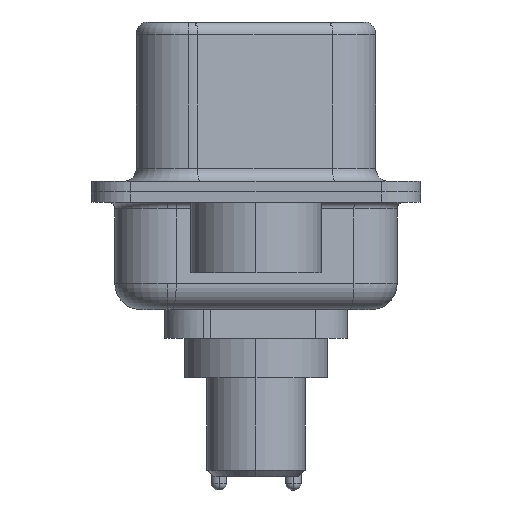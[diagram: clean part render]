
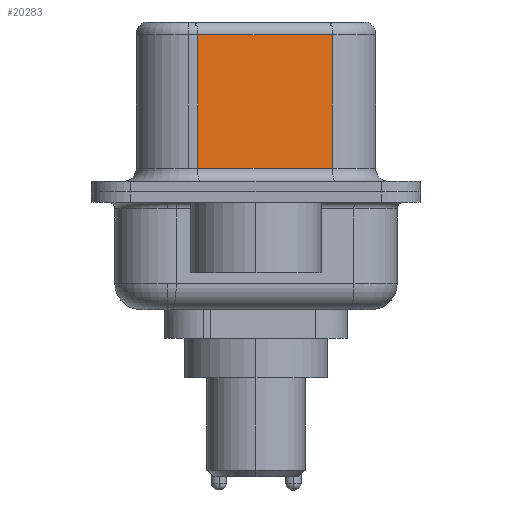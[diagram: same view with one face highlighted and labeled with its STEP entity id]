
A CAD part, left-side view. The second image highlights one B-rep face of the part: STEP entity #20283.
In plain terms, the highlighted planar face has unit normal (-0.985, -0.174, 0).
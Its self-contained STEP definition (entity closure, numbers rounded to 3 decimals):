
#166 = DIRECTION ( 'NONE',  ( 0., 0., -1. ) ) ;
#474 = VERTEX_POINT ( 'NONE', #5944 ) ;
#1858 = EDGE_CURVE ( 'NONE', #18986, #15144, #6978, .T. ) ;
#3460 = LINE ( 'NONE', #5739, #17208 ) ;
#3616 = DIRECTION ( 'NONE',  ( -0.174, 0.985, 0. ) ) ;
#3842 = VECTOR ( 'NONE', #9684, 1000. ) ;
#4164 = EDGE_LOOP ( 'NONE', ( #8791, #6228, #21408, #9122 ) ) ;
#4368 = DIRECTION ( 'NONE',  ( -0.174, 0.985, 0. ) ) ;
#5328 = CARTESIAN_POINT ( 'NONE',  ( 4.58, -2.927, 0.9 ) ) ;
#5566 = VECTOR ( 'NONE', #166, 1000. ) ;
#5739 = CARTESIAN_POINT ( 'NONE',  ( 4.58, -2.927, 6.02 ) ) ;
#5944 = CARTESIAN_POINT ( 'NONE',  ( 4.58, -2.927, 6.02 ) ) ;
#6083 = LINE ( 'NONE', #11162, #5566 ) ;
#6118 = DIRECTION ( 'NONE',  ( 0.174, -0.985, 0. ) ) ;
#6221 = EDGE_CURVE ( 'NONE', #12866, #18986, #6083, .T. ) ;
#6228 = ORIENTED_EDGE ( 'NONE', *, *, #8336, .T. ) ;
#6978 = LINE ( 'NONE', #5328, #21207 ) ;
#7474 = AXIS2_PLACEMENT_3D ( 'NONE', #18474, #13536, #3616 ) ;
#8262 = LINE ( 'NONE', #16238, #3842 ) ;
#8336 = EDGE_CURVE ( 'NONE', #474, #12866, #3460, .T. ) ;
#8791 = ORIENTED_EDGE ( 'NONE', *, *, #11874, .F. ) ;
#9122 = ORIENTED_EDGE ( 'NONE', *, *, #1858, .T. ) ;
#9684 = DIRECTION ( 'NONE',  ( 0., 0., -1. ) ) ;
#10158 = PLANE ( 'NONE',  #7474 ) ;
#11162 = CARTESIAN_POINT ( 'NONE',  ( 3.67, 2.233, 6.52 ) ) ;
#11874 = EDGE_CURVE ( 'NONE', #474, #15144, #8262, .T. ) ;
#11933 = CARTESIAN_POINT ( 'NONE',  ( 3.67, 2.233, 0.9 ) ) ;
#12866 = VERTEX_POINT ( 'NONE', #19332 ) ;
#13536 = DIRECTION ( 'NONE',  ( 0.985, 0.174, 0. ) ) ;
#13761 = CARTESIAN_POINT ( 'NONE',  ( 4.58, -2.927, 0.9 ) ) ;
#15144 = VERTEX_POINT ( 'NONE', #13761 ) ;
#16044 = FACE_OUTER_BOUND ( 'NONE', #4164, .T. ) ;
#16238 = CARTESIAN_POINT ( 'NONE',  ( 4.58, -2.927, 6.52 ) ) ;
#17208 = VECTOR ( 'NONE', #4368, 1000. ) ;
#18474 = CARTESIAN_POINT ( 'NONE',  ( 4.58, -2.927, 6.52 ) ) ;
#18986 = VERTEX_POINT ( 'NONE', #11933 ) ;
#19332 = CARTESIAN_POINT ( 'NONE',  ( 3.67, 2.233, 6.02 ) ) ;
#20283 = ADVANCED_FACE ( 'NONE', ( #16044 ), #10158, .F. ) ;
#21207 = VECTOR ( 'NONE', #6118, 1000. ) ;
#21408 = ORIENTED_EDGE ( 'NONE', *, *, #6221, .T. ) ;
